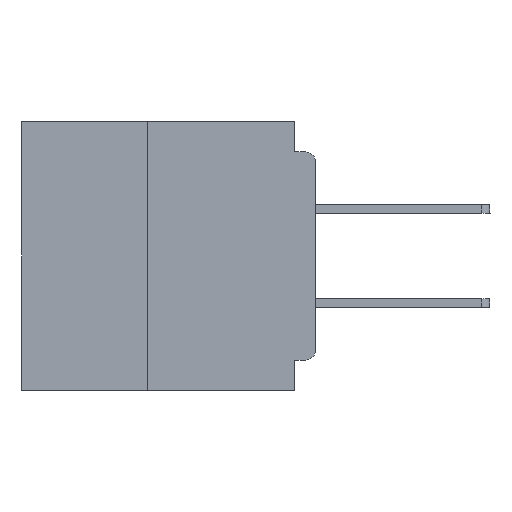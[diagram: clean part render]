
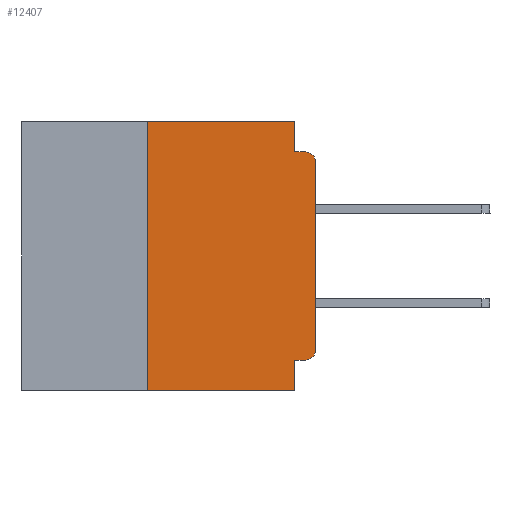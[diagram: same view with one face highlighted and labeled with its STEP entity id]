
A CAD part, left-side view. The second image highlights one B-rep face of the part: STEP entity #12407.
In plain terms, the highlighted planar face has unit normal (-1, 0, 0).
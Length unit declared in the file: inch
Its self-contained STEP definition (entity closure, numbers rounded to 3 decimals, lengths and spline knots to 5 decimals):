
#707 = DIRECTION ( 'NONE',  ( 0., 0., -1. ) ) ;
#1185 = VERTEX_POINT ( 'NONE', #21687 ) ;
#2179 = AXIS2_PLACEMENT_3D ( 'NONE', #10311, #47068, #15559 ) ;
#3275 = LINE ( 'NONE', #36478, #41897 ) ;
#4202 = ORIENTED_EDGE ( 'NONE', *, *, #51776, .T. ) ;
#5415 = CARTESIAN_POINT ( 'NONE',  ( 0., 0.015, -0.355 ) ) ;
#6016 = CIRCLE ( 'NONE', #2179, 0.015 ) ;
#8564 = CARTESIAN_POINT ( 'NONE',  ( 0., 0.031, -0.355 ) ) ;
#10311 = CARTESIAN_POINT ( 'NONE',  ( 0., 0.015, -0.34 ) ) ;
#11390 = AXIS2_PLACEMENT_3D ( 'NONE', #47886, #32181, #707 ) ;
#12407 = ADVANCED_FACE ( 'NONE', ( #17564 ), #26882, .F. ) ;
#12798 = EDGE_CURVE ( 'NONE', #38265, #39273, #45486, .T. ) ;
#15559 = DIRECTION ( 'NONE',  ( 0., 0., -1. ) ) ;
#16818 = ORIENTED_EDGE ( 'NONE', *, *, #19230, .F. ) ;
#17564 = FACE_OUTER_BOUND ( 'NONE', #38668, .T. ) ;
#18362 = VERTEX_POINT ( 'NONE', #26945 ) ;
#19230 = EDGE_CURVE ( 'NONE', #48779, #31330, #40966, .T. ) ;
#19556 = ORIENTED_EDGE ( 'NONE', *, *, #63970, .F. ) ;
#19628 = CARTESIAN_POINT ( 'NONE',  ( 0., 0.031, -0.045 ) ) ;
#20497 = ORIENTED_EDGE ( 'NONE', *, *, #46574, .T. ) ;
#21687 = CARTESIAN_POINT ( 'NONE',  ( 0., 0.25, -0.4 ) ) ;
#22138 = DIRECTION ( 'NONE',  ( 0., 0., 1. ) ) ;
#22201 = CARTESIAN_POINT ( 'NONE',  ( 0., 0.015, -0.06 ) ) ;
#22798 = ORIENTED_EDGE ( 'NONE', *, *, #33866, .F. ) ;
#23273 = LINE ( 'NONE', #36697, #35650 ) ;
#25645 = ORIENTED_EDGE ( 'NONE', *, *, #43247, .T. ) ;
#25703 = LINE ( 'NONE', #45022, #39733 ) ;
#26882 = PLANE ( 'NONE',  #11390 ) ;
#26945 = CARTESIAN_POINT ( 'NONE',  ( 0., 0., -0.34 ) ) ;
#26961 = VECTOR ( 'NONE', #63915, 39.37008 ) ;
#27117 = CARTESIAN_POINT ( 'NONE',  ( 0., 0.031, -0.4 ) ) ;
#27505 = DIRECTION ( 'NONE',  ( 0., 0., -1. ) ) ;
#27975 = VERTEX_POINT ( 'NONE', #36421 ) ;
#29270 = CARTESIAN_POINT ( 'NONE',  ( 0., 0.437, -0.4 ) ) ;
#29909 = CARTESIAN_POINT ( 'NONE',  ( 0., 0.031, 0. ) ) ;
#31330 = VERTEX_POINT ( 'NONE', #29909 ) ;
#31456 = VECTOR ( 'NONE', #66581, 39.37008 ) ;
#32181 = DIRECTION ( 'NONE',  ( 1., 0., 0. ) ) ;
#33726 = LINE ( 'NONE', #29270, #61740 ) ;
#33792 = ORIENTED_EDGE ( 'NONE', *, *, #12798, .F. ) ;
#33866 = EDGE_CURVE ( 'NONE', #31330, #38265, #23273, .T. ) ;
#35153 = CARTESIAN_POINT ( 'NONE',  ( 0., 0., -0.045 ) ) ;
#35604 = EDGE_CURVE ( 'NONE', #1185, #27975, #33726, .T. ) ;
#35650 = VECTOR ( 'NONE', #43516, 39.37008 ) ;
#36421 = CARTESIAN_POINT ( 'NONE',  ( 0., 0.031, -0.4 ) ) ;
#36478 = CARTESIAN_POINT ( 'NONE',  ( 0., 0., -0.355 ) ) ;
#36697 = CARTESIAN_POINT ( 'NONE',  ( 0., 0.031, 0. ) ) ;
#37802 = CARTESIAN_POINT ( 'NONE',  ( 0., 0., -0.06 ) ) ;
#38265 = VERTEX_POINT ( 'NONE', #19628 ) ;
#38668 = EDGE_LOOP ( 'NONE', ( #20497, #4202, #33792, #22798, #16818, #40311, #51431, #19556, #40768, #25645 ) ) ;
#39273 = VERTEX_POINT ( 'NONE', #39989 ) ;
#39716 = VECTOR ( 'NONE', #22138, 39.37008 ) ;
#39733 = VECTOR ( 'NONE', #44806, 39.37008 ) ;
#39989 = CARTESIAN_POINT ( 'NONE',  ( 0., 0.015, -0.045 ) ) ;
#40311 = ORIENTED_EDGE ( 'NONE', *, *, #55676, .F. ) ;
#40768 = ORIENTED_EDGE ( 'NONE', *, *, #52152, .F. ) ;
#40966 = LINE ( 'NONE', #65667, #50047 ) ;
#41754 = DIRECTION ( 'NONE',  ( 0., 1., 0. ) ) ;
#41897 = VECTOR ( 'NONE', #41754, 39.37008 ) ;
#42428 = VERTEX_POINT ( 'NONE', #5415 ) ;
#43128 = CARTESIAN_POINT ( 'NONE',  ( 0., 0., 0. ) ) ;
#43247 = EDGE_CURVE ( 'NONE', #42428, #18362, #6016, .T. ) ;
#43516 = DIRECTION ( 'NONE',  ( 0., 0., -1. ) ) ;
#44322 = VERTEX_POINT ( 'NONE', #8564 ) ;
#44599 = DIRECTION ( 'NONE',  ( 0., -1., 0. ) ) ;
#44806 = DIRECTION ( 'NONE',  ( 0., 0., 1. ) ) ;
#45022 = CARTESIAN_POINT ( 'NONE',  ( 0., 0.25, -0.4 ) ) ;
#45420 = CARTESIAN_POINT ( 'NONE',  ( 0., 0.25, 0. ) ) ;
#45486 = LINE ( 'NONE', #35153, #31456 ) ;
#46556 = VERTEX_POINT ( 'NONE', #37802 ) ;
#46574 = EDGE_CURVE ( 'NONE', #18362, #46556, #53771, .T. ) ;
#47068 = DIRECTION ( 'NONE',  ( -1., 0., 0. ) ) ;
#47886 = CARTESIAN_POINT ( 'NONE',  ( 0., 0.437, 0. ) ) ;
#48779 = VERTEX_POINT ( 'NONE', #45420 ) ;
#50047 = VECTOR ( 'NONE', #44599, 39.37008 ) ;
#51431 = ORIENTED_EDGE ( 'NONE', *, *, #35604, .T. ) ;
#51776 = EDGE_CURVE ( 'NONE', #46556, #39273, #64950, .T. ) ;
#52152 = EDGE_CURVE ( 'NONE', #42428, #44322, #3275, .T. ) ;
#53386 = LINE ( 'NONE', #27117, #26961 ) ;
#53771 = LINE ( 'NONE', #43128, #39716 ) ;
#54583 = AXIS2_PLACEMENT_3D ( 'NONE', #22201, #59107, #27505 ) ;
#55590 = DIRECTION ( 'NONE',  ( 0., -1., 0. ) ) ;
#55676 = EDGE_CURVE ( 'NONE', #1185, #48779, #25703, .T. ) ;
#59107 = DIRECTION ( 'NONE',  ( -1., 0., 0. ) ) ;
#61740 = VECTOR ( 'NONE', #55590, 39.37008 ) ;
#63915 = DIRECTION ( 'NONE',  ( 0., 0., -1. ) ) ;
#63970 = EDGE_CURVE ( 'NONE', #44322, #27975, #53386, .T. ) ;
#64950 = CIRCLE ( 'NONE', #54583, 0.015 ) ;
#65667 = CARTESIAN_POINT ( 'NONE',  ( 0., 0.437, 0. ) ) ;
#66581 = DIRECTION ( 'NONE',  ( 0., -1., 0. ) ) ;
